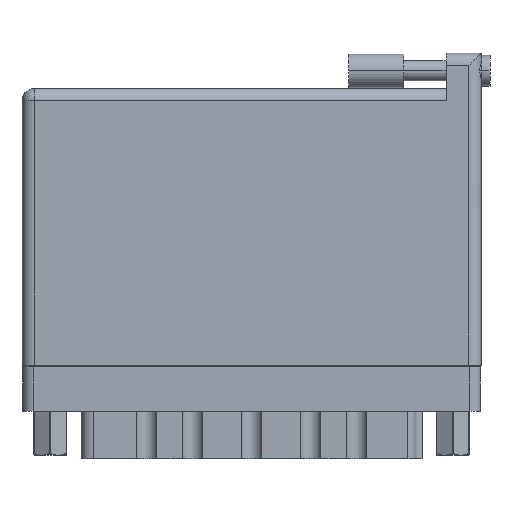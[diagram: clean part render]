
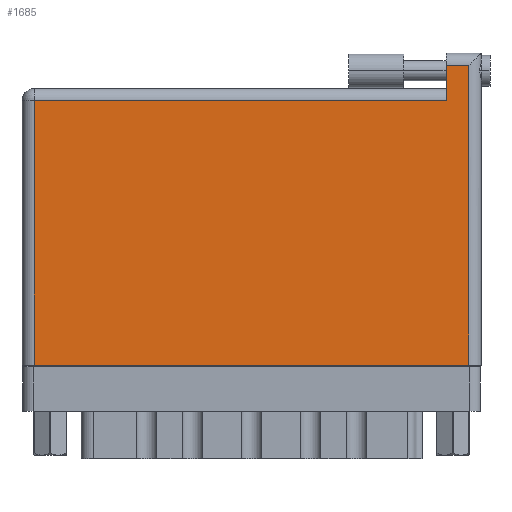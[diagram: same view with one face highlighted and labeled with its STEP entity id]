
A CAD part, front view. The second image highlights one B-rep face of the part: STEP entity #1685.
In plain terms, the highlighted face is planar.
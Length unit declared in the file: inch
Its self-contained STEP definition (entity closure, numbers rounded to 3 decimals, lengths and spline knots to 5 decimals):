
#392 = VERTEX_POINT ( 'NONE', #28552 ) ;
#461 = LINE ( 'NONE', #15792, #16886 ) ;
#551 = CARTESIAN_POINT ( 'NONE',  ( 0., 1.496, 0. ) ) ;
#644 = ORIENTED_EDGE ( 'NONE', *, *, #23811, .T. ) ;
#845 = CARTESIAN_POINT ( 'NONE',  ( 2.53, 0., 0. ) ) ;
#1685 = ADVANCED_FACE ( 'NONE', ( #31054 ), #45252, .F. ) ;
#2290 = CARTESIAN_POINT ( 'NONE',  ( 0., 1.566, 0. ) ) ;
#2694 = DIRECTION ( 'NONE',  ( 0., 1., 0. ) ) ;
#3920 = CARTESIAN_POINT ( 'NONE',  ( 2.403, 1.496, 0. ) ) ;
#4866 = EDGE_LOOP ( 'NONE', ( #53716, #644, #40149, #21414, #25708, #31197 ) ) ;
#8179 = VERTEX_POINT ( 'NONE', #42937 ) ;
#8486 = CARTESIAN_POINT ( 'NONE',  ( 0.07, 0., 0. ) ) ;
#11855 = VECTOR ( 'NONE', #23810, 39.37008 ) ;
#12341 = CARTESIAN_POINT ( 'NONE',  ( 2.53, 1.766, 0. ) ) ;
#12845 = VERTEX_POINT ( 'NONE', #8486 ) ;
#13708 = CARTESIAN_POINT ( 'NONE',  ( 2.53, 1.696, 0. ) ) ;
#15007 = AXIS2_PLACEMENT_3D ( 'NONE', #2290, #35792, #20717 ) ;
#15792 = CARTESIAN_POINT ( 'NONE',  ( 0.07, 0., 0. ) ) ;
#16661 = EDGE_CURVE ( 'NONE', #49602, #8179, #55534, .T. ) ;
#16886 = VECTOR ( 'NONE', #20589, 39.37008 ) ;
#20490 = EDGE_CURVE ( 'NONE', #8179, #12845, #461, .T. ) ;
#20589 = DIRECTION ( 'NONE',  ( 0., -1., 0. ) ) ;
#20717 = DIRECTION ( 'NONE',  ( -1., 0., 0. ) ) ;
#21414 = ORIENTED_EDGE ( 'NONE', *, *, #59892, .T. ) ;
#21936 = LINE ( 'NONE', #12341, #61721 ) ;
#22831 = VERTEX_POINT ( 'NONE', #13708 ) ;
#23471 = VERTEX_POINT ( 'NONE', #845 ) ;
#23810 = DIRECTION ( 'NONE',  ( 0., -1., 0. ) ) ;
#23811 = EDGE_CURVE ( 'NONE', #23471, #22831, #21936, .T. ) ;
#25372 = CARTESIAN_POINT ( 'NONE',  ( 0., 0., 0. ) ) ;
#25708 = ORIENTED_EDGE ( 'NONE', *, *, #16661, .T. ) ;
#26077 = LINE ( 'NONE', #42486, #11855 ) ;
#28552 = CARTESIAN_POINT ( 'NONE',  ( 2.403, 1.696, 0. ) ) ;
#31054 = FACE_OUTER_BOUND ( 'NONE', #4866, .T. ) ;
#31197 = ORIENTED_EDGE ( 'NONE', *, *, #20490, .T. ) ;
#31932 = EDGE_CURVE ( 'NONE', #22831, #392, #56163, .T. ) ;
#33673 = DIRECTION ( 'NONE',  ( -1., 0., 0. ) ) ;
#35792 = DIRECTION ( 'NONE',  ( 0., 0., -1. ) ) ;
#40149 = ORIENTED_EDGE ( 'NONE', *, *, #31932, .T. ) ;
#41227 = VECTOR ( 'NONE', #43290, 39.37008 ) ;
#42486 = CARTESIAN_POINT ( 'NONE',  ( 2.403, 1.766, 0. ) ) ;
#42937 = CARTESIAN_POINT ( 'NONE',  ( 0.07, 1.496, 0. ) ) ;
#43290 = DIRECTION ( 'NONE',  ( -1., 0., 0. ) ) ;
#43402 = VECTOR ( 'NONE', #33673, 39.37008 ) ;
#45252 = PLANE ( 'NONE',  #15007 ) ;
#49602 = VERTEX_POINT ( 'NONE', #3920 ) ;
#52847 = CARTESIAN_POINT ( 'NONE',  ( 0., 1.696, 0. ) ) ;
#53716 = ORIENTED_EDGE ( 'NONE', *, *, #56164, .T. ) ;
#55205 = LINE ( 'NONE', #25372, #55975 ) ;
#55534 = LINE ( 'NONE', #551, #41227 ) ;
#55975 = VECTOR ( 'NONE', #58960, 39.37008 ) ;
#56163 = LINE ( 'NONE', #52847, #43402 ) ;
#56164 = EDGE_CURVE ( 'NONE', #12845, #23471, #55205, .T. ) ;
#58960 = DIRECTION ( 'NONE',  ( 1., 0., 0. ) ) ;
#59892 = EDGE_CURVE ( 'NONE', #392, #49602, #26077, .T. ) ;
#61721 = VECTOR ( 'NONE', #2694, 39.37008 ) ;
